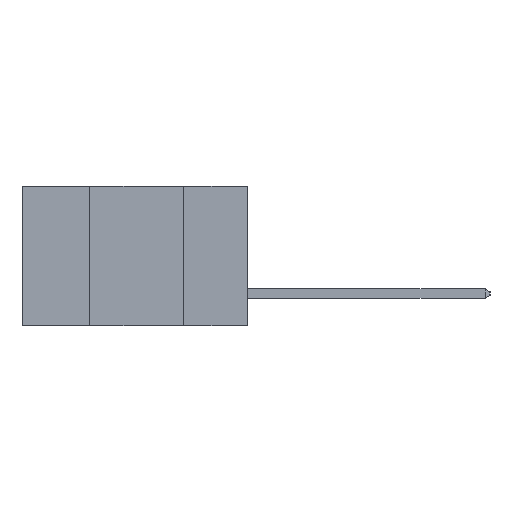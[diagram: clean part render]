
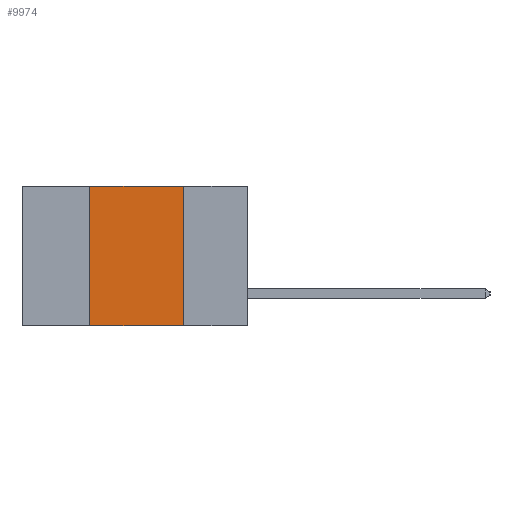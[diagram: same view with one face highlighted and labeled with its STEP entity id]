
A CAD part, left-side view. The second image highlights one B-rep face of the part: STEP entity #9974.
In plain terms, the highlighted planar face has unit normal (-1, 0, 0).
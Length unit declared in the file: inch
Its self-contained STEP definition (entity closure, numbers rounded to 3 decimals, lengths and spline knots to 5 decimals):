
#25 = EDGE_CURVE ( 'NONE', #1829, #3449, #3899, .T. ) ;
#276 = VECTOR ( 'NONE', #4079, 39.37008 ) ;
#403 = CARTESIAN_POINT ( 'NONE',  ( 0., 0.42, -0.37 ) ) ;
#499 = VERTEX_POINT ( 'NONE', #12119 ) ;
#1829 = VERTEX_POINT ( 'NONE', #5700 ) ;
#2250 = CARTESIAN_POINT ( 'NONE',  ( 0., 0.6, -0.37 ) ) ;
#2602 = EDGE_LOOP ( 'NONE', ( #10027, #10182, #10313, #10514 ) ) ;
#2772 = AXIS2_PLACEMENT_3D ( 'NONE', #13692, #14712, #8192 ) ;
#2993 = VECTOR ( 'NONE', #9228, 39.37008 ) ;
#3449 = VERTEX_POINT ( 'NONE', #7325 ) ;
#3899 = LINE ( 'NONE', #5283, #276 ) ;
#4079 = DIRECTION ( 'NONE',  ( 0., 0., -1. ) ) ;
#5283 = CARTESIAN_POINT ( 'NONE',  ( 0., 0.17, -0.37 ) ) ;
#5571 = CARTESIAN_POINT ( 'NONE',  ( 0., 0.42, -0.37 ) ) ;
#5700 = CARTESIAN_POINT ( 'NONE',  ( 0., 0.17, 0. ) ) ;
#5936 = PLANE ( 'NONE',  #2772 ) ;
#6433 = VECTOR ( 'NONE', #6713, 39.37008 ) ;
#6713 = DIRECTION ( 'NONE',  ( 0., 0., 1. ) ) ;
#7325 = CARTESIAN_POINT ( 'NONE',  ( 0., 0.17, -0.37 ) ) ;
#7482 = EDGE_CURVE ( 'NONE', #11626, #3449, #12139, .T. ) ;
#8192 = DIRECTION ( 'NONE',  ( 0., 0., -1. ) ) ;
#9228 = DIRECTION ( 'NONE',  ( 0., -1., 0. ) ) ;
#9570 = DIRECTION ( 'NONE',  ( 0., -1., 0. ) ) ;
#9736 = VECTOR ( 'NONE', #9570, 39.37008 ) ;
#9974 = ADVANCED_FACE ( 'NONE', ( #10144 ), #5936, .F. ) ;
#10027 = ORIENTED_EDGE ( 'NONE', *, *, #25, .F. ) ;
#10144 = FACE_OUTER_BOUND ( 'NONE', #2602, .T. ) ;
#10182 = ORIENTED_EDGE ( 'NONE', *, *, #12686, .F. ) ;
#10313 = ORIENTED_EDGE ( 'NONE', *, *, #10503, .F. ) ;
#10503 = EDGE_CURVE ( 'NONE', #11626, #499, #12378, .T. ) ;
#10514 = ORIENTED_EDGE ( 'NONE', *, *, #7482, .T. ) ;
#11626 = VERTEX_POINT ( 'NONE', #403 ) ;
#11754 = CARTESIAN_POINT ( 'NONE',  ( 0., 0.6, 0. ) ) ;
#12119 = CARTESIAN_POINT ( 'NONE',  ( 0., 0.42, 0. ) ) ;
#12139 = LINE ( 'NONE', #2250, #2993 ) ;
#12378 = LINE ( 'NONE', #5571, #6433 ) ;
#12683 = LINE ( 'NONE', #11754, #9736 ) ;
#12686 = EDGE_CURVE ( 'NONE', #499, #1829, #12683, .T. ) ;
#13692 = CARTESIAN_POINT ( 'NONE',  ( 0., 0.6, 0. ) ) ;
#14712 = DIRECTION ( 'NONE',  ( 1., 0., 0. ) ) ;
